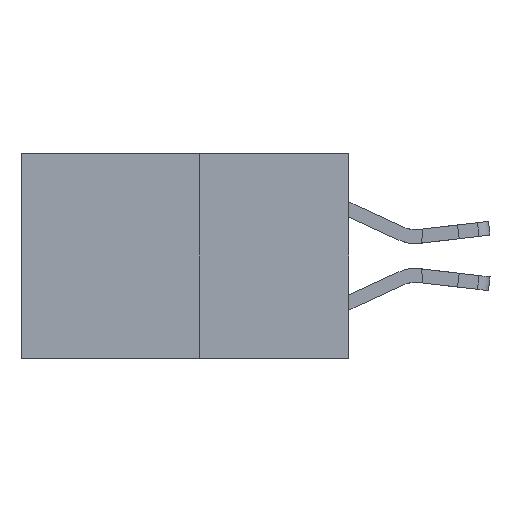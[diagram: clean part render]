
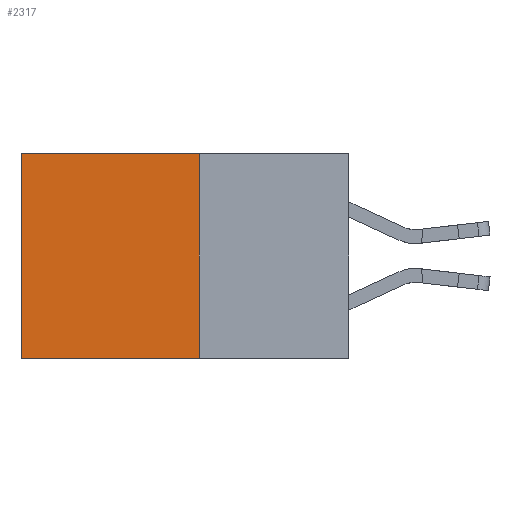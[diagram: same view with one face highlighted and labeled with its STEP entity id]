
A CAD part, left-side view. The second image highlights one B-rep face of the part: STEP entity #2317.
In plain terms, the highlighted planar face has unit normal (-1, 0, 0).
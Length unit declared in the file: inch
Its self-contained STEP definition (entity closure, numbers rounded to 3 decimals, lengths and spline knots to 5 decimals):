
#142 = ORIENTED_EDGE ( 'NONE', *, *, #6857, .F. ) ;
#212 = VERTEX_POINT ( 'NONE', #4523 ) ;
#276 = CARTESIAN_POINT ( 'NONE',  ( 0.277, 0.27, -0.37 ) ) ;
#279 = LINE ( 'NONE', #10375, #12316 ) ;
#680 = FACE_OUTER_BOUND ( 'NONE', #1101, .T. ) ;
#1101 = EDGE_LOOP ( 'NONE', ( #2649, #3021, #142, #3398 ) ) ;
#1340 = AXIS2_PLACEMENT_3D ( 'NONE', #14103, #10836, #2484 ) ;
#1717 = EDGE_CURVE ( 'NONE', #212, #12034, #279, .T. ) ;
#2317 = ADVANCED_FACE ( 'NONE', ( #680 ), #11775, .F. ) ;
#2484 = DIRECTION ( 'NONE',  ( 0., 0., -1. ) ) ;
#2649 = ORIENTED_EDGE ( 'NONE', *, *, #4586, .T. ) ;
#2696 = VERTEX_POINT ( 'NONE', #4983 ) ;
#3021 = ORIENTED_EDGE ( 'NONE', *, *, #8606, .F. ) ;
#3398 = ORIENTED_EDGE ( 'NONE', *, *, #1717, .T. ) ;
#4523 = CARTESIAN_POINT ( 'NONE',  ( 0.277, 0.27, 0. ) ) ;
#4586 = EDGE_CURVE ( 'NONE', #12034, #11706, #9256, .T. ) ;
#4983 = CARTESIAN_POINT ( 'NONE',  ( 0.277, 0.27, -0.37 ) ) ;
#6076 = LINE ( 'NONE', #14581, #14685 ) ;
#6353 = CARTESIAN_POINT ( 'NONE',  ( 0.277, 0.59, -0.37 ) ) ;
#6857 = EDGE_CURVE ( 'NONE', #212, #2696, #6076, .T. ) ;
#7053 = DIRECTION ( 'NONE',  ( 0., 1., 0. ) ) ;
#8606 = EDGE_CURVE ( 'NONE', #2696, #11706, #14472, .T. ) ;
#9256 = LINE ( 'NONE', #12291, #14748 ) ;
#9730 = DIRECTION ( 'NONE',  ( 0., 1., 0. ) ) ;
#10375 = CARTESIAN_POINT ( 'NONE',  ( 0.277, 0.27, 0. ) ) ;
#10836 = DIRECTION ( 'NONE',  ( 1., 0., 0. ) ) ;
#11706 = VERTEX_POINT ( 'NONE', #6353 ) ;
#11775 = PLANE ( 'NONE',  #1340 ) ;
#12034 = VERTEX_POINT ( 'NONE', #13837 ) ;
#12193 = DIRECTION ( 'NONE',  ( 0., 0., -1. ) ) ;
#12291 = CARTESIAN_POINT ( 'NONE',  ( 0.277, 0.59, -0.37 ) ) ;
#12316 = VECTOR ( 'NONE', #7053, 39.37008 ) ;
#13000 = VECTOR ( 'NONE', #9730, 39.37008 ) ;
#13519 = DIRECTION ( 'NONE',  ( 0., 0., -1. ) ) ;
#13837 = CARTESIAN_POINT ( 'NONE',  ( 0.277, 0.59, 0. ) ) ;
#14103 = CARTESIAN_POINT ( 'NONE',  ( 0.277, 0.27, -0.37 ) ) ;
#14472 = LINE ( 'NONE', #276, #13000 ) ;
#14581 = CARTESIAN_POINT ( 'NONE',  ( 0.277, 0.27, -0.37 ) ) ;
#14685 = VECTOR ( 'NONE', #13519, 39.37008 ) ;
#14748 = VECTOR ( 'NONE', #12193, 39.37008 ) ;
